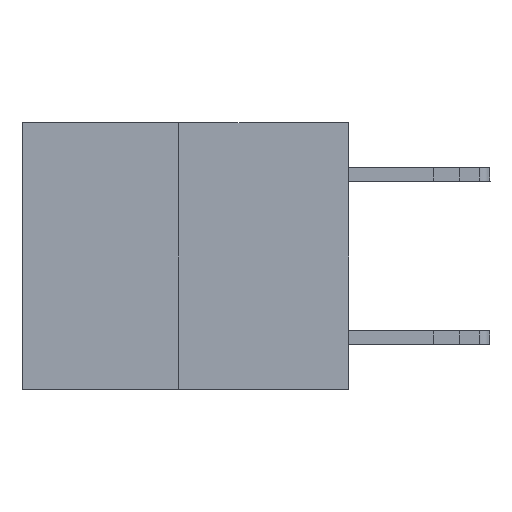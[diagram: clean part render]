
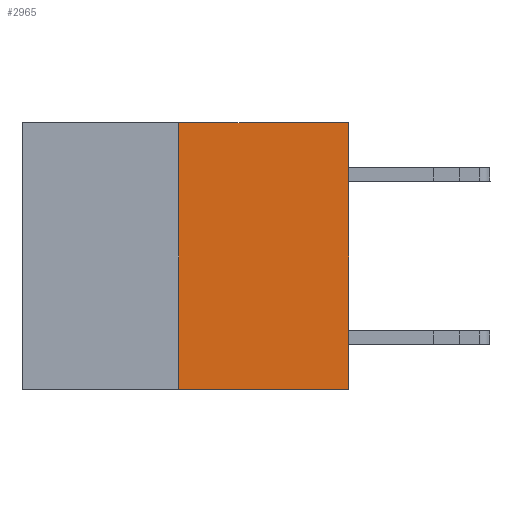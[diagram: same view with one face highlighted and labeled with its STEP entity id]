
A CAD part, left-side view. The second image highlights one B-rep face of the part: STEP entity #2965.
In plain terms, the highlighted planar face has unit normal (-1, 0, 0).
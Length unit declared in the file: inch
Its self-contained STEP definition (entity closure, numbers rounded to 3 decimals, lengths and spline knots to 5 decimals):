
#174 = VERTEX_POINT ( 'NONE', #19580 ) ;
#1736 = VERTEX_POINT ( 'NONE', #15359 ) ;
#1812 = VECTOR ( 'NONE', #29264, 39.37008 ) ;
#1971 = VECTOR ( 'NONE', #19823, 39.37008 ) ;
#2024 = DIRECTION ( 'NONE',  ( 0., 0., 1. ) ) ;
#2806 = CARTESIAN_POINT ( 'NONE',  ( 0., 0.6, 0. ) ) ;
#2965 = ADVANCED_FACE ( 'NONE', ( #22672 ), #29628, .F. ) ;
#3045 = VERTEX_POINT ( 'NONE', #20973 ) ;
#4053 = CARTESIAN_POINT ( 'NONE',  ( 0., 0.6, 0. ) ) ;
#4208 = EDGE_CURVE ( 'NONE', #3045, #174, #25150, .T. ) ;
#5811 = DIRECTION ( 'NONE',  ( 0., 0., 1. ) ) ;
#5970 = EDGE_CURVE ( 'NONE', #174, #24982, #15505, .T. ) ;
#6500 = DIRECTION ( 'NONE',  ( 0., 0., -1. ) ) ;
#8205 = EDGE_LOOP ( 'NONE', ( #25473, #28463, #25112, #18403 ) ) ;
#11308 = CARTESIAN_POINT ( 'NONE',  ( 0., 0., 0. ) ) ;
#14716 = AXIS2_PLACEMENT_3D ( 'NONE', #4053, #20451, #6500 ) ;
#15359 = CARTESIAN_POINT ( 'NONE',  ( 0., 0., -0.49 ) ) ;
#15505 = LINE ( 'NONE', #2806, #1971 ) ;
#15818 = LINE ( 'NONE', #11308, #18013 ) ;
#16080 = EDGE_CURVE ( 'NONE', #1736, #24982, #15818, .T. ) ;
#17236 = CARTESIAN_POINT ( 'NONE',  ( 0., 0.6, -0.49 ) ) ;
#18013 = VECTOR ( 'NONE', #2024, 39.37008 ) ;
#18403 = ORIENTED_EDGE ( 'NONE', *, *, #5970, .F. ) ;
#18932 = VECTOR ( 'NONE', #5811, 39.37008 ) ;
#19580 = CARTESIAN_POINT ( 'NONE',  ( 0., 0.312, 0. ) ) ;
#19648 = CARTESIAN_POINT ( 'NONE',  ( 0., 0.312, -0.49 ) ) ;
#19823 = DIRECTION ( 'NONE',  ( 0., -1., 0. ) ) ;
#20451 = DIRECTION ( 'NONE',  ( 1., 0., 0. ) ) ;
#20973 = CARTESIAN_POINT ( 'NONE',  ( 0., 0.312, -0.49 ) ) ;
#21709 = CARTESIAN_POINT ( 'NONE',  ( 0., 0., 0. ) ) ;
#22672 = FACE_OUTER_BOUND ( 'NONE', #8205, .T. ) ;
#24982 = VERTEX_POINT ( 'NONE', #21709 ) ;
#25112 = ORIENTED_EDGE ( 'NONE', *, *, #16080, .T. ) ;
#25150 = LINE ( 'NONE', #19648, #18932 ) ;
#25473 = ORIENTED_EDGE ( 'NONE', *, *, #4208, .F. ) ;
#26457 = EDGE_CURVE ( 'NONE', #3045, #1736, #28131, .T. ) ;
#28131 = LINE ( 'NONE', #17236, #1812 ) ;
#28463 = ORIENTED_EDGE ( 'NONE', *, *, #26457, .T. ) ;
#29264 = DIRECTION ( 'NONE',  ( 0., -1., 0. ) ) ;
#29628 = PLANE ( 'NONE',  #14716 ) ;
